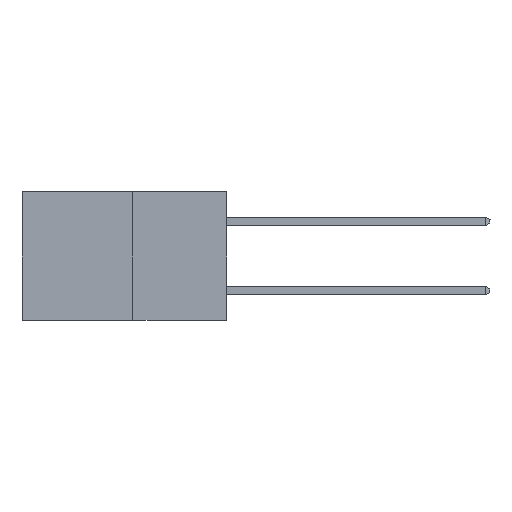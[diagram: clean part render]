
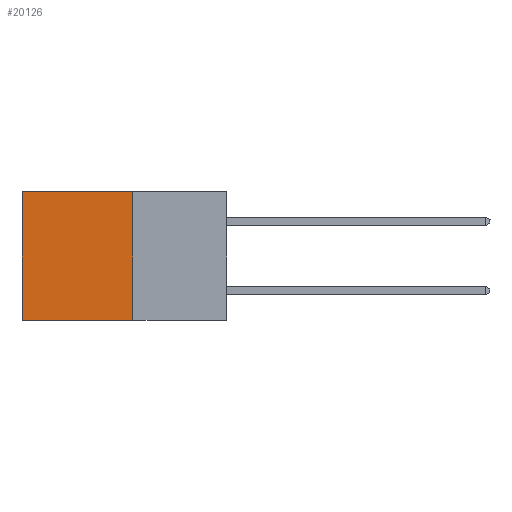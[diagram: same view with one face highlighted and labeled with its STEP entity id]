
A CAD part, left-side view. The second image highlights one B-rep face of the part: STEP entity #20126.
In plain terms, the highlighted planar face has unit normal (-1, 0, 0).
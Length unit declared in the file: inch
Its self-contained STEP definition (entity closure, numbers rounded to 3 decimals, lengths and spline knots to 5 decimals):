
#180 = VECTOR ( 'NONE', #18593, 39.37008 ) ;
#1692 = CARTESIAN_POINT ( 'NONE',  ( 0.277, 0.27, 0. ) ) ;
#1736 = EDGE_LOOP ( 'NONE', ( #7337, #10866, #11189, #2023 ) ) ;
#2023 = ORIENTED_EDGE ( 'NONE', *, *, #2889, .T. ) ;
#2420 = LINE ( 'NONE', #17820, #17905 ) ;
#2889 = EDGE_CURVE ( 'NONE', #5025, #18256, #11526, .T. ) ;
#3608 = CARTESIAN_POINT ( 'NONE',  ( 0.277, 0.27, -0.37 ) ) ;
#3609 = CARTESIAN_POINT ( 'NONE',  ( 0.277, 0.27, -0.37 ) ) ;
#3994 = VECTOR ( 'NONE', #13760, 39.37008 ) ;
#5025 = VERTEX_POINT ( 'NONE', #1692 ) ;
#5229 = CARTESIAN_POINT ( 'NONE',  ( 0.277, 0.59, -0.37 ) ) ;
#5266 = AXIS2_PLACEMENT_3D ( 'NONE', #3608, #19729, #7646 ) ;
#5525 = VERTEX_POINT ( 'NONE', #3609 ) ;
#5758 = DIRECTION ( 'NONE',  ( 0., 0., -1. ) ) ;
#6156 = VECTOR ( 'NONE', #17321, 39.37008 ) ;
#7337 = ORIENTED_EDGE ( 'NONE', *, *, #13910, .T. ) ;
#7646 = DIRECTION ( 'NONE',  ( 0., 0., -1. ) ) ;
#8201 = EDGE_CURVE ( 'NONE', #5025, #5525, #2420, .T. ) ;
#8571 = VERTEX_POINT ( 'NONE', #5229 ) ;
#10579 = FACE_OUTER_BOUND ( 'NONE', #1736, .T. ) ;
#10866 = ORIENTED_EDGE ( 'NONE', *, *, #16254, .F. ) ;
#11189 = ORIENTED_EDGE ( 'NONE', *, *, #8201, .F. ) ;
#11526 = LINE ( 'NONE', #18308, #6156 ) ;
#13760 = DIRECTION ( 'NONE',  ( 0., 1., 0. ) ) ;
#13910 = EDGE_CURVE ( 'NONE', #18256, #8571, #16398, .T. ) ;
#14113 = LINE ( 'NONE', #17787, #3994 ) ;
#16003 = CARTESIAN_POINT ( 'NONE',  ( 0.277, 0.59, 0. ) ) ;
#16254 = EDGE_CURVE ( 'NONE', #5525, #8571, #14113, .T. ) ;
#16398 = LINE ( 'NONE', #16581, #180 ) ;
#16581 = CARTESIAN_POINT ( 'NONE',  ( 0.277, 0.59, -0.37 ) ) ;
#17321 = DIRECTION ( 'NONE',  ( 0., 1., 0. ) ) ;
#17712 = PLANE ( 'NONE',  #5266 ) ;
#17787 = CARTESIAN_POINT ( 'NONE',  ( 0.277, 0.27, -0.37 ) ) ;
#17820 = CARTESIAN_POINT ( 'NONE',  ( 0.277, 0.27, -0.37 ) ) ;
#17905 = VECTOR ( 'NONE', #5758, 39.37008 ) ;
#18256 = VERTEX_POINT ( 'NONE', #16003 ) ;
#18308 = CARTESIAN_POINT ( 'NONE',  ( 0.277, 0.27, 0. ) ) ;
#18593 = DIRECTION ( 'NONE',  ( 0., 0., -1. ) ) ;
#19729 = DIRECTION ( 'NONE',  ( 1., 0., 0. ) ) ;
#20126 = ADVANCED_FACE ( 'NONE', ( #10579 ), #17712, .F. ) ;
